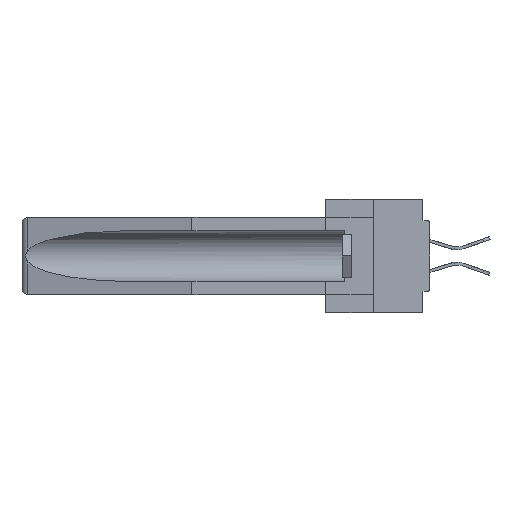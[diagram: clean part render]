
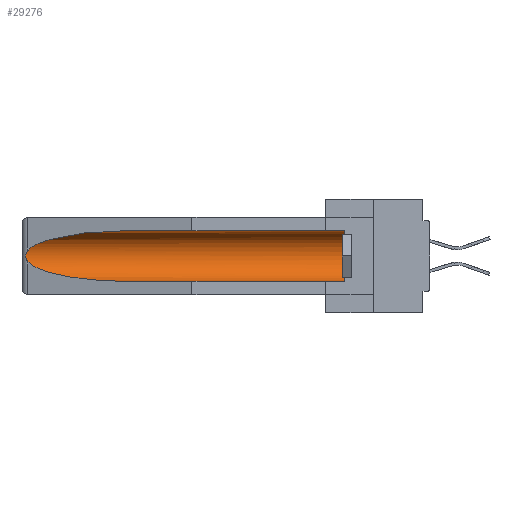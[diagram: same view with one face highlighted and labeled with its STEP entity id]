
A CAD part, left-side view. The second image highlights one B-rep face of the part: STEP entity #29276.
In plain terms, the highlighted cylindrical face has radius 2.857 mm (diameter 5.715 mm), a partial arc.
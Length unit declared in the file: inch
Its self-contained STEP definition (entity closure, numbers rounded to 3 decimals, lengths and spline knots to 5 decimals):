
#327 = ORIENTED_EDGE ( 'NONE', *, *, #44007, .T. ) ;
#2845 = CARTESIAN_POINT ( 'NONE',  ( 0.25451, 1.48313, -0.24835 ) ) ;
#3100 = DIRECTION ( 'NONE',  ( 0., -1., 0. ) ) ;
#3131 = VERTEX_POINT ( 'NONE', #32588 ) ;
#3986 = AXIS2_PLACEMENT_3D ( 'NONE', #9776, #3100, #33843 ) ;
#4157 = CARTESIAN_POINT ( 'NONE',  ( 0.2675, 1.53308, -0.16763 ) ) ;
#4291 = ORIENTED_EDGE ( 'NONE', *, *, #23564, .T. ) ;
#4308 = CARTESIAN_POINT ( 'NONE',  ( 0.2673, 1.5327, -0.16383 ) ) ;
#6349 = CARTESIAN_POINT ( 'NONE',  ( 0.21114, 1.30732, -0.284 ) ) ;
#7383 = CARTESIAN_POINT ( 'NONE',  ( 0.26654, 1.53092, -0.15636 ) ) ;
#7663 = CARTESIAN_POINT ( 'NONE',  ( 0.26537, 1.52718, -0.14972 ) ) ;
#8138 = CARTESIAN_POINT ( 'NONE',  ( 0.26537, 1.52718, -0.14972 ) ) ;
#8287 = ORIENTED_EDGE ( 'NONE', *, *, #8921, .T. ) ;
#8915 = VECTOR ( 'NONE', #12490, 39.37008 ) ;
#8921 = EDGE_CURVE ( 'NONE', #16541, #32238, #12188, .T. ) ;
#9164 = CYLINDRICAL_SURFACE ( 'NONE', #43893, 0.1125 ) ;
#9776 = CARTESIAN_POINT ( 'NONE',  ( 0.155, 0.126, -0.1715 ) ) ;
#10697 = CARTESIAN_POINT ( 'NONE',  ( 0.26597, 1.52961, -0.15275 ) ) ;
#10839 = CARTESIAN_POINT ( 'NONE',  ( 0.2673, 1.53269, -0.17917 ) ) ;
#10999 = EDGE_CURVE ( 'NONE', #32238, #14934, #19108, .T. ) ;
#11110 = ORIENTED_EDGE ( 'NONE', *, *, #29622, .F. ) ;
#11502 = CIRCLE ( 'NONE', #3986, 0.1125 ) ;
#12188 = LINE ( 'NONE', #29604, #8915 ) ;
#12490 = DIRECTION ( 'NONE',  ( 0., 1., 0. ) ) ;
#13326 = CARTESIAN_POINT ( 'NONE',  ( 0.155, 1.07973, -0.284 ) ) ;
#14183 = CARTESIAN_POINT ( 'NONE',  ( 0.26597, 1.5296, -0.19026 ) ) ;
#14652 = FACE_OUTER_BOUND ( 'NONE', #15970, .T. ) ;
#14934 = VERTEX_POINT ( 'NONE', #15599 ) ;
#15599 = CARTESIAN_POINT ( 'NONE',  ( 0.26537, 1.52718, -0.14972 ) ) ;
#15970 = EDGE_LOOP ( 'NONE', ( #28943, #31821, #4291, #11110, #327, #8287 ) ) ;
#16541 = VERTEX_POINT ( 'NONE', #35237 ) ;
#17636 = CARTESIAN_POINT ( 'NONE',  ( 0.26537, 1.52718, -0.19328 ) ) ;
#18284 =( BOUNDED_CURVE ( )  B_SPLINE_CURVE ( 3, ( #33591, #2845, #6349, #13326 ),
 .UNSPECIFIED., .F., .T. ) 
 B_SPLINE_CURVE_WITH_KNOTS ( ( 4, 4 ),
 ( 0.1948, 1.5708 ),
 .UNSPECIFIED. ) 
 CURVE ( )  GEOMETRIC_REPRESENTATION_ITEM ( )  RATIONAL_B_SPLINE_CURVE ( ( 1., 0.848, 0.848, 1. ) ) 
 REPRESENTATION_ITEM ( '' )  );
#19005 = CARTESIAN_POINT ( 'NONE',  ( 0.155, -0.30754, -0.1715 ) ) ;
#19108 =( BOUNDED_CURVE ( )  B_SPLINE_CURVE ( 3, ( #28583, #42751, #32499, #8138 ),
 .UNSPECIFIED., .F., .F. ) 
 B_SPLINE_CURVE_WITH_KNOTS ( ( 4, 4 ),
 ( 4.71239, 6.08839 ),
 .UNSPECIFIED. ) 
 CURVE ( )  GEOMETRIC_REPRESENTATION_ITEM ( )  RATIONAL_B_SPLINE_CURVE ( ( 1., 0.848, 0.848, 1. ) ) 
 REPRESENTATION_ITEM ( '' )  );
#19611 = VERTEX_POINT ( 'NONE', #24890 ) ;
#22893 = DIRECTION ( 'NONE',  ( 0., 0., 1. ) ) ;
#23564 = EDGE_CURVE ( 'NONE', #3131, #29251, #18284, .T. ) ;
#24890 = CARTESIAN_POINT ( 'NONE',  ( 0.155, 0.126, -0.284 ) ) ;
#28299 = CARTESIAN_POINT ( 'NONE',  ( 0.2675, 1.53308, -0.17534 ) ) ;
#28583 = CARTESIAN_POINT ( 'NONE',  ( 0.155, 1.07973, -0.059 ) ) ;
#28943 = ORIENTED_EDGE ( 'NONE', *, *, #10999, .T. ) ;
#29019 = CARTESIAN_POINT ( 'NONE',  ( 0.155, -0.30754, -0.284 ) ) ;
#29140 = LINE ( 'NONE', #29019, #33950 ) ;
#29251 = VERTEX_POINT ( 'NONE', #39899 ) ;
#29276 = ADVANCED_FACE ( 'NONE', ( #14652 ), #9164, .F. ) ;
#29604 = CARTESIAN_POINT ( 'NONE',  ( 0.155, -0.30754, -0.059 ) ) ;
#29622 = EDGE_CURVE ( 'NONE', #19611, #29251, #29140, .T. ) ;
#31821 = ORIENTED_EDGE ( 'NONE', *, *, #33127, .T. ) ;
#32238 = VERTEX_POINT ( 'NONE', #34862 ) ;
#32325 = DIRECTION ( 'NONE',  ( 0., 1., 0. ) ) ;
#32499 = CARTESIAN_POINT ( 'NONE',  ( 0.25451, 1.48313, -0.09465 ) ) ;
#32588 = CARTESIAN_POINT ( 'NONE',  ( 0.26537, 1.52718, -0.19328 ) ) ;
#33127 = EDGE_CURVE ( 'NONE', #14934, #3131, #35626, .T. ) ;
#33591 = CARTESIAN_POINT ( 'NONE',  ( 0.26537, 1.52718, -0.19328 ) ) ;
#33843 = DIRECTION ( 'NONE',  ( 0., 0., 1. ) ) ;
#33950 = VECTOR ( 'NONE', #32325, 39.37008 ) ;
#34742 = CARTESIAN_POINT ( 'NONE',  ( 0.26655, 1.53094, -0.18657 ) ) ;
#34862 = CARTESIAN_POINT ( 'NONE',  ( 0.155, 1.07973, -0.059 ) ) ;
#35237 = CARTESIAN_POINT ( 'NONE',  ( 0.155, 0.126, -0.059 ) ) ;
#35626 = B_SPLINE_CURVE_WITH_KNOTS ( 'NONE', 3,
 ( #7663, #10697, #7383, #4308, #4157, #28299, #10839, #34742, #14183, #17636 ),
 .UNSPECIFIED., .F., .F.,
 ( 4, 2, 2, 2, 4 ),
 ( 0., 0.00029, 0.00058, 0.00087, 0.00117 ),
 .UNSPECIFIED. ) ;
#39899 = CARTESIAN_POINT ( 'NONE',  ( 0.155, 1.07973, -0.284 ) ) ;
#42751 = CARTESIAN_POINT ( 'NONE',  ( 0.21114, 1.30732, -0.059 ) ) ;
#43510 = DIRECTION ( 'NONE',  ( 0., 1., 0. ) ) ;
#43893 = AXIS2_PLACEMENT_3D ( 'NONE', #19005, #43510, #22893 ) ;
#44007 = EDGE_CURVE ( 'NONE', #19611, #16541, #11502, .T. ) ;
